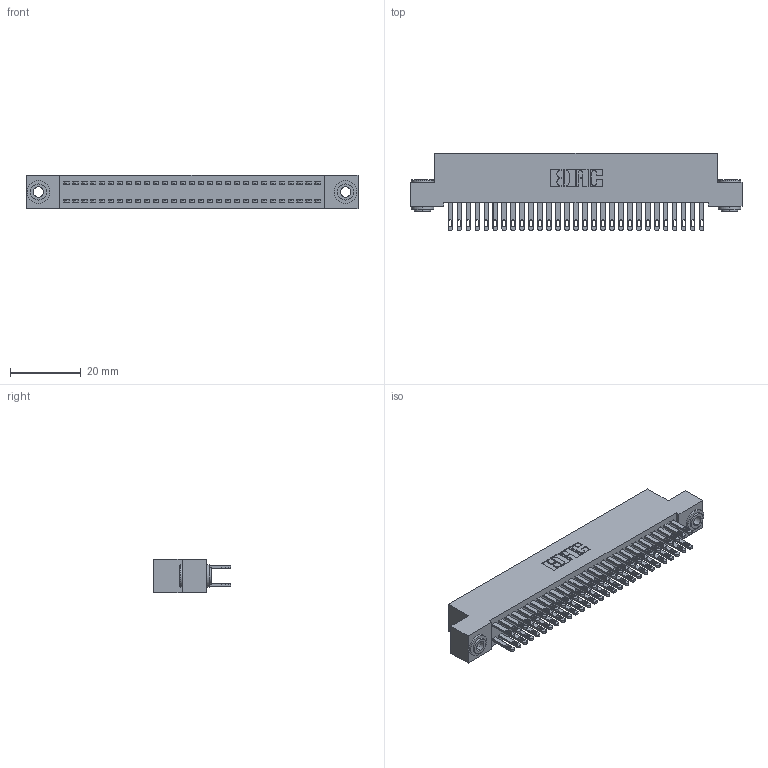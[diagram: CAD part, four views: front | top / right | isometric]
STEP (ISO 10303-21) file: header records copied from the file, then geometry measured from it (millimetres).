
FILE_DESCRIPTION (( 'STEP AP203' ), '1' );
FILE_NAME ('892-058-500-203.STEP', '2020-09-21T19:02:35', ( '' ), ( '' ), 'SwSTEP 2.0', 'SolidWorks 2020', '' );
FILE_SCHEMA (( 'CONFIG_CONTROL_DESIGN' ));
Length unit declared in the file: inch
Products named in the file (4): 345-292-001_345-293-100; 342-250-002_345-250-002-102; 892-058-500-203; 842 Part_.156 TH
Assembly tree (61 placements, depth 2):
  892-058-500-203
    842 Part_.156 TH
    345-292-001_345-293-100  x58
    342-250-002_345-250-002-102  x2
Bounding box: 93.98 x 21.85 x 9.4 mm (x, y, z)
Volume: 8582.6 mm3; surface area: 14419.4 mm2
Topology: 61 solids, 61 shells, 2932 faces, 8901 edges, 5930 vertices
Faces by surface type: plane 1816, cylinder 1108, cone 8
Entity records: 20786 total; most frequent: CARTESIAN_POINT 3433, ORIENTED_EDGE 3362, DIRECTION 2991, EDGE_CURVE 1681, VECTOR 1525, LINE 1525, VERTEX_POINT 1118, AXIS2_PLACEMENT_3D 733
